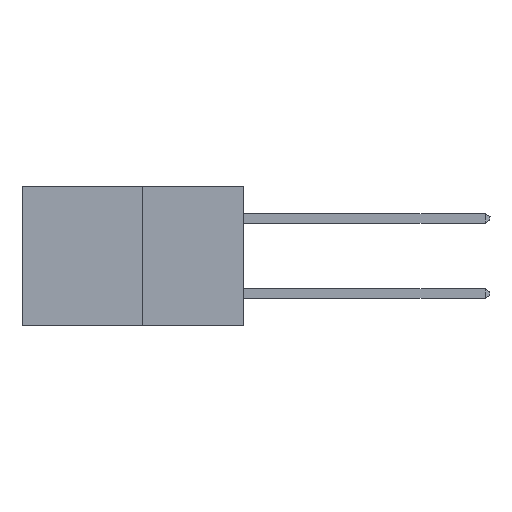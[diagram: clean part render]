
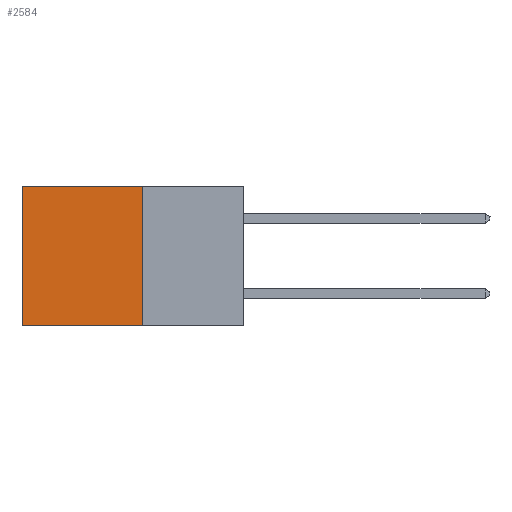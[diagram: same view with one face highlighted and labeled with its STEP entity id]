
A CAD part, left-side view. The second image highlights one B-rep face of the part: STEP entity #2584.
In plain terms, the highlighted planar face has unit normal (-1, 0, 0).
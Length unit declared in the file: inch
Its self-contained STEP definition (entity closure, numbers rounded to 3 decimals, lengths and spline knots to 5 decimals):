
#1109 = FACE_OUTER_BOUND ( 'NONE', #15395, .T. ) ;
#1543 = CARTESIAN_POINT ( 'NONE',  ( 0.277, 0.27, -0.37 ) ) ;
#1981 = VERTEX_POINT ( 'NONE', #12668 ) ;
#2584 = ADVANCED_FACE ( 'NONE', ( #1109 ), #5686, .F. ) ;
#2735 = AXIS2_PLACEMENT_3D ( 'NONE', #5750, #9129, #14702 ) ;
#3125 = CARTESIAN_POINT ( 'NONE',  ( 0.277, 0.59, -0.37 ) ) ;
#3400 = VECTOR ( 'NONE', #13692, 39.37008 ) ;
#3409 = VERTEX_POINT ( 'NONE', #3125 ) ;
#3952 = VERTEX_POINT ( 'NONE', #7485 ) ;
#3955 = LINE ( 'NONE', #7203, #14666 ) ;
#3996 = LINE ( 'NONE', #4637, #17419 ) ;
#4066 = ORIENTED_EDGE ( 'NONE', *, *, #8859, .T. ) ;
#4637 = CARTESIAN_POINT ( 'NONE',  ( 0.277, 0.27, -0.37 ) ) ;
#4871 = VECTOR ( 'NONE', #12779, 39.37008 ) ;
#5307 = LINE ( 'NONE', #1543, #4871 ) ;
#5686 = PLANE ( 'NONE',  #2735 ) ;
#5750 = CARTESIAN_POINT ( 'NONE',  ( 0.277, 0.27, -0.37 ) ) ;
#5871 = DIRECTION ( 'NONE',  ( 0., 1., 0. ) ) ;
#5905 = EDGE_CURVE ( 'NONE', #3952, #3409, #11297, .T. ) ;
#7203 = CARTESIAN_POINT ( 'NONE',  ( 0.277, 0.27, 0. ) ) ;
#7485 = CARTESIAN_POINT ( 'NONE',  ( 0.277, 0.59, 0. ) ) ;
#7850 = CARTESIAN_POINT ( 'NONE',  ( 0.277, 0.27, 0. ) ) ;
#8858 = DIRECTION ( 'NONE',  ( 0., 1., 0. ) ) ;
#8859 = EDGE_CURVE ( 'NONE', #13565, #3952, #3955, .T. ) ;
#9129 = DIRECTION ( 'NONE',  ( 1., 0., 0. ) ) ;
#11085 = ORIENTED_EDGE ( 'NONE', *, *, #15907, .F. ) ;
#11297 = LINE ( 'NONE', #13739, #3400 ) ;
#12180 = ORIENTED_EDGE ( 'NONE', *, *, #5905, .T. ) ;
#12668 = CARTESIAN_POINT ( 'NONE',  ( 0.277, 0.27, -0.37 ) ) ;
#12779 = DIRECTION ( 'NONE',  ( 0., 0., -1. ) ) ;
#13463 = ORIENTED_EDGE ( 'NONE', *, *, #16032, .F. ) ;
#13565 = VERTEX_POINT ( 'NONE', #7850 ) ;
#13692 = DIRECTION ( 'NONE',  ( 0., 0., -1. ) ) ;
#13739 = CARTESIAN_POINT ( 'NONE',  ( 0.277, 0.59, -0.37 ) ) ;
#14666 = VECTOR ( 'NONE', #5871, 39.37008 ) ;
#14702 = DIRECTION ( 'NONE',  ( 0., 0., -1. ) ) ;
#15395 = EDGE_LOOP ( 'NONE', ( #12180, #13463, #11085, #4066 ) ) ;
#15907 = EDGE_CURVE ( 'NONE', #13565, #1981, #5307, .T. ) ;
#16032 = EDGE_CURVE ( 'NONE', #1981, #3409, #3996, .T. ) ;
#17419 = VECTOR ( 'NONE', #8858, 39.37008 ) ;
